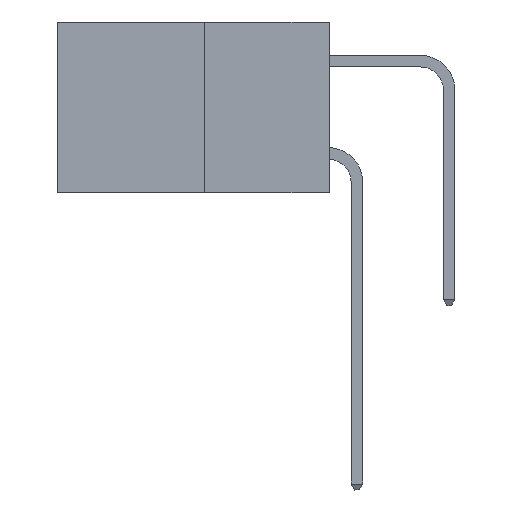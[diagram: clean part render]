
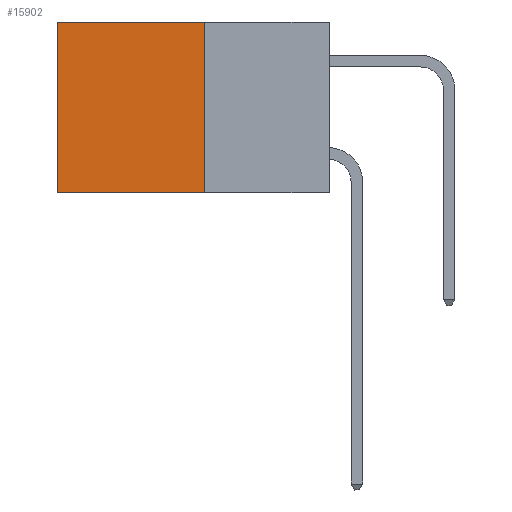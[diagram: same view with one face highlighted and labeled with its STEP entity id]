
A CAD part, left-side view. The second image highlights one B-rep face of the part: STEP entity #15902.
In plain terms, the highlighted planar face has unit normal (-1, 0, 0).
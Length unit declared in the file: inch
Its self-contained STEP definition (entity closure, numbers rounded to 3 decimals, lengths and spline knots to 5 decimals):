
#26 = EDGE_CURVE ( 'NONE', #1415, #3470, #9879, .T. ) ;
#377 = EDGE_CURVE ( 'NONE', #14171, #1485, #4284, .T. ) ;
#524 = VECTOR ( 'NONE', #6932, 39.37008 ) ;
#1331 = VECTOR ( 'NONE', #9859, 39.37008 ) ;
#1415 = VERTEX_POINT ( 'NONE', #10933 ) ;
#1485 = VERTEX_POINT ( 'NONE', #7535 ) ;
#1552 = CARTESIAN_POINT ( 'NONE',  ( 0.277, 0.59, -0.37 ) ) ;
#1836 = PLANE ( 'NONE',  #6290 ) ;
#2798 = LINE ( 'NONE', #14700, #16654 ) ;
#2821 = EDGE_LOOP ( 'NONE', ( #3512, #4919, #11726, #7952 ) ) ;
#3470 = VERTEX_POINT ( 'NONE', #9428 ) ;
#3512 = ORIENTED_EDGE ( 'NONE', *, *, #13877, .T. ) ;
#4284 = LINE ( 'NONE', #9297, #524 ) ;
#4699 = DIRECTION ( 'NONE',  ( 1., 0., 0. ) ) ;
#4919 = ORIENTED_EDGE ( 'NONE', *, *, #26, .F. ) ;
#5831 = VECTOR ( 'NONE', #11773, 39.37008 ) ;
#6290 = AXIS2_PLACEMENT_3D ( 'NONE', #12995, #4699, #14402 ) ;
#6346 = CARTESIAN_POINT ( 'NONE',  ( 0.277, 0.27, 0. ) ) ;
#6932 = DIRECTION ( 'NONE',  ( 0., 1., 0. ) ) ;
#7535 = CARTESIAN_POINT ( 'NONE',  ( 0.277, 0.59, 0. ) ) ;
#7952 = ORIENTED_EDGE ( 'NONE', *, *, #377, .T. ) ;
#8299 = LINE ( 'NONE', #1552, #1331 ) ;
#9297 = CARTESIAN_POINT ( 'NONE',  ( 0.277, 0.27, 0. ) ) ;
#9428 = CARTESIAN_POINT ( 'NONE',  ( 0.277, 0.59, -0.37 ) ) ;
#9527 = EDGE_CURVE ( 'NONE', #14171, #1415, #2798, .T. ) ;
#9859 = DIRECTION ( 'NONE',  ( 0., 0., -1. ) ) ;
#9879 = LINE ( 'NONE', #13534, #5831 ) ;
#10933 = CARTESIAN_POINT ( 'NONE',  ( 0.277, 0.27, -0.37 ) ) ;
#11511 = FACE_OUTER_BOUND ( 'NONE', #2821, .T. ) ;
#11726 = ORIENTED_EDGE ( 'NONE', *, *, #9527, .F. ) ;
#11773 = DIRECTION ( 'NONE',  ( 0., 1., 0. ) ) ;
#12995 = CARTESIAN_POINT ( 'NONE',  ( 0.277, 0.27, -0.37 ) ) ;
#13364 = DIRECTION ( 'NONE',  ( 0., 0., -1. ) ) ;
#13534 = CARTESIAN_POINT ( 'NONE',  ( 0.277, 0.27, -0.37 ) ) ;
#13877 = EDGE_CURVE ( 'NONE', #1485, #3470, #8299, .T. ) ;
#14171 = VERTEX_POINT ( 'NONE', #6346 ) ;
#14402 = DIRECTION ( 'NONE',  ( 0., 0., -1. ) ) ;
#14700 = CARTESIAN_POINT ( 'NONE',  ( 0.277, 0.27, -0.37 ) ) ;
#15902 = ADVANCED_FACE ( 'NONE', ( #11511 ), #1836, .F. ) ;
#16654 = VECTOR ( 'NONE', #13364, 39.37008 ) ;
